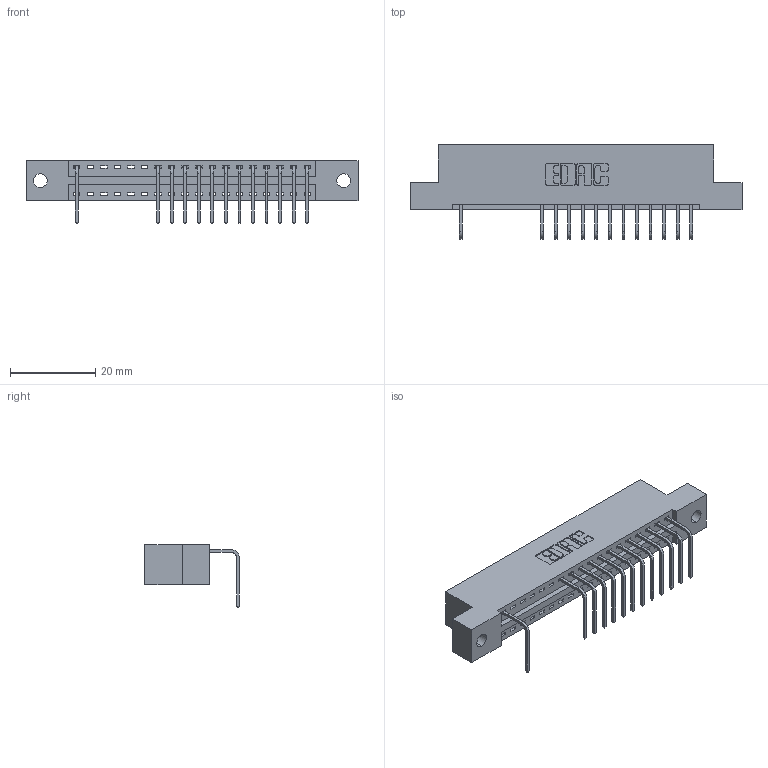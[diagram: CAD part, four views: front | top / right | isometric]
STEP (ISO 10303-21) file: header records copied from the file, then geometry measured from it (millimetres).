
FILE_DESCRIPTION (( 'STEP AP203' ), '1' );
FILE_NAME ('346-018-558-102.STEP', '2018-08-20T08:45:07', ( '' ), ( '' ), 'SwSTEP 2.0', 'SolidWorks 2016', '' );
FILE_SCHEMA (( 'CONFIG_CONTROL_DESIGN' ));
Length unit declared in the file: inch
Products named in the file (3): 346 Part_Flush Mounting Lugs - 0.128 Dia; 345-292-001_558 Tail - 2; 346-018-558-102
Assembly tree (14 placements, depth 2):
  346-018-558-102
    346 Part_Flush Mounting Lugs - 0.128 Dia
    345-292-001_558 Tail - 2  x13
Bounding box: 77.72 x 22.16 x 14.73 mm (x, y, z)
Volume: 7224 mm3; surface area: 8449.6 mm2
Topology: 14 solids, 14 shells, 962 faces, 2905 edges, 1918 vertices
Faces by surface type: plane 672, cylinder 290
Entity records: 14329 total; most frequent: CARTESIAN_POINT 2493, ORIENTED_EDGE 2450, DIRECTION 2223, EDGE_CURVE 1225, LINE 1021, VECTOR 1021, VERTEX_POINT 814, AXIS2_PLACEMENT_3D 601
